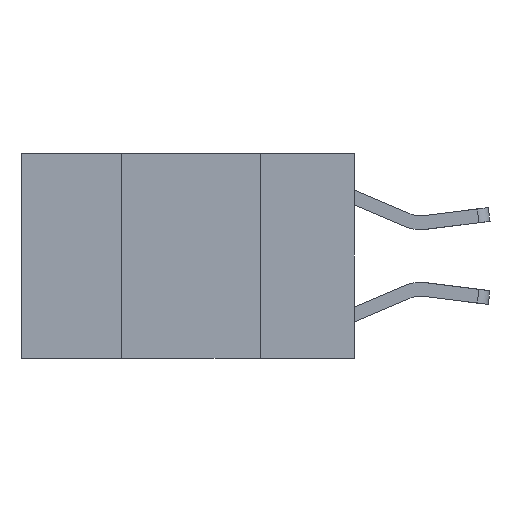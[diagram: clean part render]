
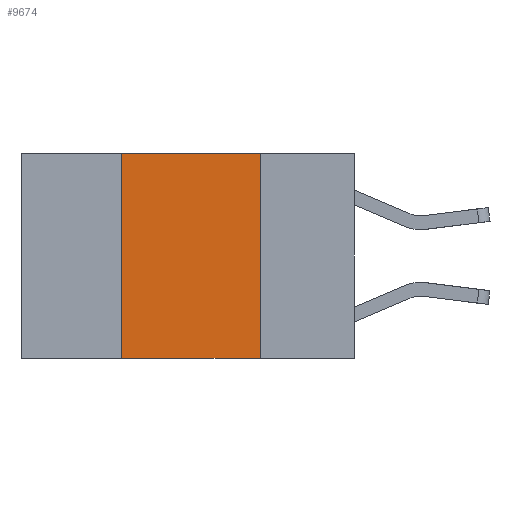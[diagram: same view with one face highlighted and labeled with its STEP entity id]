
A CAD part, left-side view. The second image highlights one B-rep face of the part: STEP entity #9674.
In plain terms, the highlighted planar face has unit normal (-1, 0, 0).
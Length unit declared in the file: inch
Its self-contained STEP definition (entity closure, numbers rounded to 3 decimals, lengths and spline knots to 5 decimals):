
#103 = VERTEX_POINT ( 'NONE', #10262 ) ;
#321 = EDGE_CURVE ( 'NONE', #8153, #103, #9498, .T. ) ;
#331 = PLANE ( 'NONE',  #5728 ) ;
#1225 = EDGE_LOOP ( 'NONE', ( #2452, #3752, #7341, #10509 ) ) ;
#1691 = CARTESIAN_POINT ( 'NONE',  ( 0., 0.6, 0. ) ) ;
#1824 = VECTOR ( 'NONE', #11845, 39.37008 ) ;
#2148 = VECTOR ( 'NONE', #7034, 39.37008 ) ;
#2185 = DIRECTION ( 'NONE',  ( 1., 0., 0. ) ) ;
#2415 = EDGE_CURVE ( 'NONE', #6313, #103, #5475, .T. ) ;
#2452 = ORIENTED_EDGE ( 'NONE', *, *, #321, .F. ) ;
#2683 = VECTOR ( 'NONE', #5028, 39.37008 ) ;
#2698 = VECTOR ( 'NONE', #4259, 39.37008 ) ;
#3752 = ORIENTED_EDGE ( 'NONE', *, *, #11374, .F. ) ;
#4259 = DIRECTION ( 'NONE',  ( 0., -1., 0. ) ) ;
#4911 = LINE ( 'NONE', #6115, #2148 ) ;
#5028 = DIRECTION ( 'NONE',  ( 0., 0., -1. ) ) ;
#5475 = LINE ( 'NONE', #10304, #2698 ) ;
#5728 = AXIS2_PLACEMENT_3D ( 'NONE', #7737, #2185, #8664 ) ;
#6042 = CARTESIAN_POINT ( 'NONE',  ( 0., 0.42, -0.37 ) ) ;
#6115 = CARTESIAN_POINT ( 'NONE',  ( 0., 0.42, 0. ) ) ;
#6313 = VERTEX_POINT ( 'NONE', #6042 ) ;
#7034 = DIRECTION ( 'NONE',  ( 0., 0., 1. ) ) ;
#7053 = LINE ( 'NONE', #1691, #1824 ) ;
#7341 = ORIENTED_EDGE ( 'NONE', *, *, #10471, .F. ) ;
#7737 = CARTESIAN_POINT ( 'NONE',  ( 0., 0.6, 0. ) ) ;
#8153 = VERTEX_POINT ( 'NONE', #9513 ) ;
#8513 = CARTESIAN_POINT ( 'NONE',  ( 0., 0.42, 0. ) ) ;
#8664 = DIRECTION ( 'NONE',  ( 0., 0., -1. ) ) ;
#8681 = FACE_OUTER_BOUND ( 'NONE', #1225, .T. ) ;
#9498 = LINE ( 'NONE', #10541, #2683 ) ;
#9513 = CARTESIAN_POINT ( 'NONE',  ( 0., 0.17, 0. ) ) ;
#9578 = VERTEX_POINT ( 'NONE', #8513 ) ;
#9674 = ADVANCED_FACE ( 'NONE', ( #8681 ), #331, .F. ) ;
#10262 = CARTESIAN_POINT ( 'NONE',  ( 0., 0.17, -0.37 ) ) ;
#10304 = CARTESIAN_POINT ( 'NONE',  ( 0., 0.6, -0.37 ) ) ;
#10471 = EDGE_CURVE ( 'NONE', #6313, #9578, #4911, .T. ) ;
#10509 = ORIENTED_EDGE ( 'NONE', *, *, #2415, .T. ) ;
#10541 = CARTESIAN_POINT ( 'NONE',  ( 0., 0.17, 0. ) ) ;
#11374 = EDGE_CURVE ( 'NONE', #9578, #8153, #7053, .T. ) ;
#11845 = DIRECTION ( 'NONE',  ( 0., -1., 0. ) ) ;
